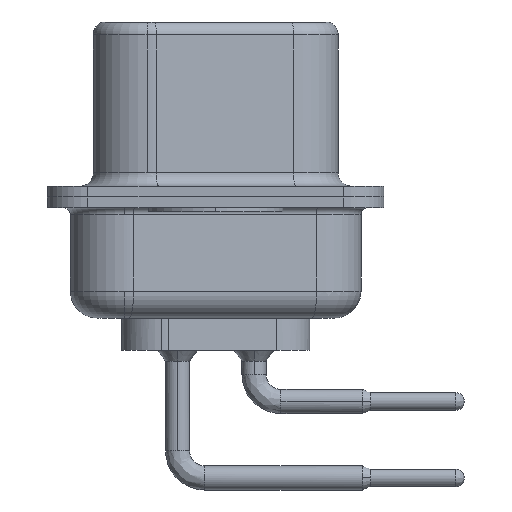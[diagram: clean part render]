
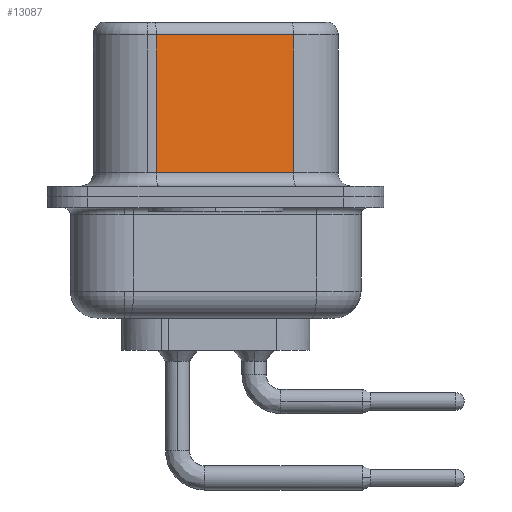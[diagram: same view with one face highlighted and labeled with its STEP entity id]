
A CAD part, left-side view. The second image highlights one B-rep face of the part: STEP entity #13087.
In plain terms, the highlighted planar face has unit normal (-0.985, -0.174, 0).
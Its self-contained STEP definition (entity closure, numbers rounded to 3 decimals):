
#692 = VERTEX_POINT ( 'NONE', #15167 ) ;
#1318 = DIRECTION ( 'NONE',  ( 0., 0., -1. ) ) ;
#2957 = DIRECTION ( 'NONE',  ( 0.174, -0.985, 0. ) ) ;
#3448 = LINE ( 'NONE', #4256, #7517 ) ;
#3695 = LINE ( 'NONE', #15553, #4150 ) ;
#4030 = CARTESIAN_POINT ( 'NONE',  ( 3.655, 2.203, 6.52 ) ) ;
#4150 = VECTOR ( 'NONE', #2957, 1000. ) ;
#4256 = CARTESIAN_POINT ( 'NONE',  ( 4.555, -2.897, 6.52 ) ) ;
#4657 = EDGE_CURVE ( 'NONE', #692, #18717, #3695, .T. ) ;
#5224 = CARTESIAN_POINT ( 'NONE',  ( 4.555, -2.897, 0.9 ) ) ;
#5423 = LINE ( 'NONE', #4030, #16966 ) ;
#6717 = ORIENTED_EDGE ( 'NONE', *, *, #13267, .T. ) ;
#7517 = VECTOR ( 'NONE', #15218, 1000. ) ;
#8087 = DIRECTION ( 'NONE',  ( 0.985, 0.174, 0. ) ) ;
#10511 = CARTESIAN_POINT ( 'NONE',  ( 4.555, -2.897, 6.02 ) ) ;
#11262 = VERTEX_POINT ( 'NONE', #13272 ) ;
#11318 = AXIS2_PLACEMENT_3D ( 'NONE', #14361, #8087, #19058 ) ;
#12261 = ORIENTED_EDGE ( 'NONE', *, *, #18852, .T. ) ;
#13025 = EDGE_LOOP ( 'NONE', ( #15261, #6717, #12261, #18903 ) ) ;
#13087 = ADVANCED_FACE ( 'NONE', ( #20045 ), #17447, .F. ) ;
#13267 = EDGE_CURVE ( 'NONE', #20040, #11262, #16529, .T. ) ;
#13272 = CARTESIAN_POINT ( 'NONE',  ( 3.655, 2.203, 6.02 ) ) ;
#13582 = DIRECTION ( 'NONE',  ( -0.174, 0.985, 0. ) ) ;
#14361 = CARTESIAN_POINT ( 'NONE',  ( 4.555, -2.897, 6.52 ) ) ;
#15167 = CARTESIAN_POINT ( 'NONE',  ( 3.655, 2.203, 0.9 ) ) ;
#15218 = DIRECTION ( 'NONE',  ( 0., 0., -1. ) ) ;
#15261 = ORIENTED_EDGE ( 'NONE', *, *, #17618, .F. ) ;
#15553 = CARTESIAN_POINT ( 'NONE',  ( 4.555, -2.897, 0.9 ) ) ;
#16529 = LINE ( 'NONE', #10511, #19791 ) ;
#16966 = VECTOR ( 'NONE', #1318, 1000. ) ;
#17447 = PLANE ( 'NONE',  #11318 ) ;
#17618 = EDGE_CURVE ( 'NONE', #20040, #18717, #3448, .T. ) ;
#18717 = VERTEX_POINT ( 'NONE', #5224 ) ;
#18852 = EDGE_CURVE ( 'NONE', #11262, #692, #5423, .T. ) ;
#18903 = ORIENTED_EDGE ( 'NONE', *, *, #4657, .T. ) ;
#19058 = DIRECTION ( 'NONE',  ( -0.174, 0.985, 0. ) ) ;
#19791 = VECTOR ( 'NONE', #13582, 1000. ) ;
#19833 = CARTESIAN_POINT ( 'NONE',  ( 4.555, -2.897, 6.02 ) ) ;
#20040 = VERTEX_POINT ( 'NONE', #19833 ) ;
#20045 = FACE_OUTER_BOUND ( 'NONE', #13025, .T. ) ;
